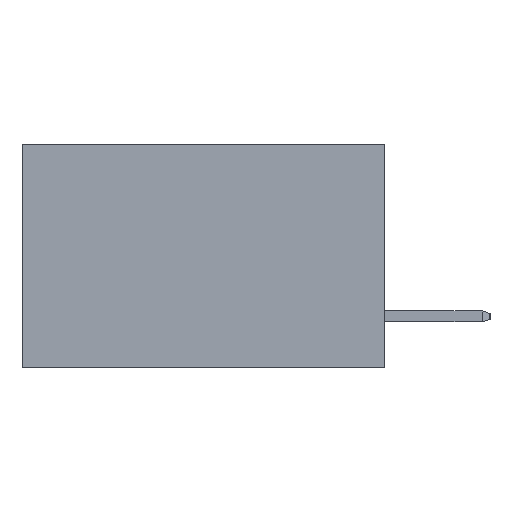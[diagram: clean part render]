
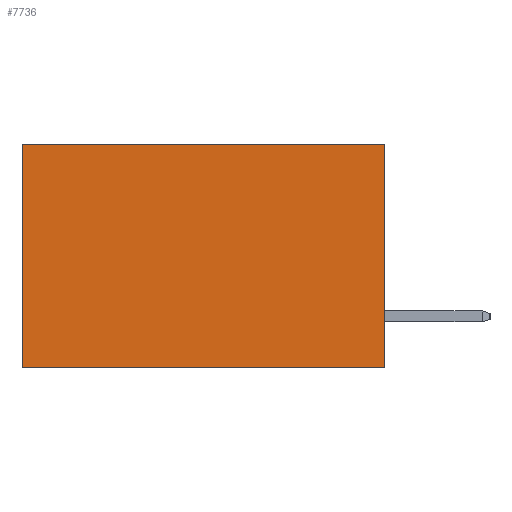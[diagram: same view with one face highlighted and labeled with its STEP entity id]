
A CAD part, left-side view. The second image highlights one B-rep face of the part: STEP entity #7736.
In plain terms, the highlighted planar face has unit normal (-1, 0, 0).
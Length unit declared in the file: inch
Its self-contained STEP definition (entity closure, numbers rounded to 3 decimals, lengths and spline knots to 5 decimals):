
#77 = VECTOR ( 'NONE', #8157, 39.37008 ) ;
#207 = DIRECTION ( 'NONE',  ( 0., 1., 0. ) ) ;
#274 = CARTESIAN_POINT ( 'NONE',  ( 0.298, 0.6, -0.37 ) ) ;
#334 = LINE ( 'NONE', #5238, #77 ) ;
#345 = FACE_OUTER_BOUND ( 'NONE', #10671, .T. ) ;
#413 = CARTESIAN_POINT ( 'NONE',  ( 0.298, 0.6, 0. ) ) ;
#710 = DIRECTION ( 'NONE',  ( 0., 0., -1. ) ) ;
#1409 = DIRECTION ( 'NONE',  ( 0., 0., -1. ) ) ;
#1528 = VERTEX_POINT ( 'NONE', #274 ) ;
#2608 = CARTESIAN_POINT ( 'NONE',  ( 0.298, 0., -0.37 ) ) ;
#2637 = DIRECTION ( 'NONE',  ( 0., 1., 0. ) ) ;
#2815 = CARTESIAN_POINT ( 'NONE',  ( 0.298, 0.6, 0. ) ) ;
#3151 = CARTESIAN_POINT ( 'NONE',  ( 0.298, 0., -0.37 ) ) ;
#3809 = CARTESIAN_POINT ( 'NONE',  ( 0.298, 0., 0. ) ) ;
#3949 = LINE ( 'NONE', #3809, #10011 ) ;
#4521 = CARTESIAN_POINT ( 'NONE',  ( 0.298, 0., 0. ) ) ;
#4615 = VECTOR ( 'NONE', #2637, 39.37008 ) ;
#4674 = EDGE_CURVE ( 'NONE', #5721, #1528, #7130, .T. ) ;
#5087 = VERTEX_POINT ( 'NONE', #7315 ) ;
#5196 = ORIENTED_EDGE ( 'NONE', *, *, #10723, .T. ) ;
#5238 = CARTESIAN_POINT ( 'NONE',  ( 0.298, 0., 0. ) ) ;
#5418 = PLANE ( 'NONE',  #6080 ) ;
#5721 = VERTEX_POINT ( 'NONE', #3151 ) ;
#6080 = AXIS2_PLACEMENT_3D ( 'NONE', #4521, #6491, #1409 ) ;
#6103 = VECTOR ( 'NONE', #710, 39.37008 ) ;
#6170 = VERTEX_POINT ( 'NONE', #413 ) ;
#6362 = EDGE_CURVE ( 'NONE', #5087, #6170, #3949, .T. ) ;
#6380 = LINE ( 'NONE', #2815, #6103 ) ;
#6491 = DIRECTION ( 'NONE',  ( 1., 0., 0. ) ) ;
#7130 = LINE ( 'NONE', #2608, #4615 ) ;
#7188 = ORIENTED_EDGE ( 'NONE', *, *, #6362, .T. ) ;
#7315 = CARTESIAN_POINT ( 'NONE',  ( 0.298, 0., 0. ) ) ;
#7736 = ADVANCED_FACE ( 'NONE', ( #345 ), #5418, .F. ) ;
#7946 = ORIENTED_EDGE ( 'NONE', *, *, #8186, .F. ) ;
#7957 = ORIENTED_EDGE ( 'NONE', *, *, #4674, .F. ) ;
#8157 = DIRECTION ( 'NONE',  ( 0., 0., -1. ) ) ;
#8186 = EDGE_CURVE ( 'NONE', #5087, #5721, #334, .T. ) ;
#10011 = VECTOR ( 'NONE', #207, 39.37008 ) ;
#10671 = EDGE_LOOP ( 'NONE', ( #5196, #7957, #7946, #7188 ) ) ;
#10723 = EDGE_CURVE ( 'NONE', #6170, #1528, #6380, .T. ) ;
